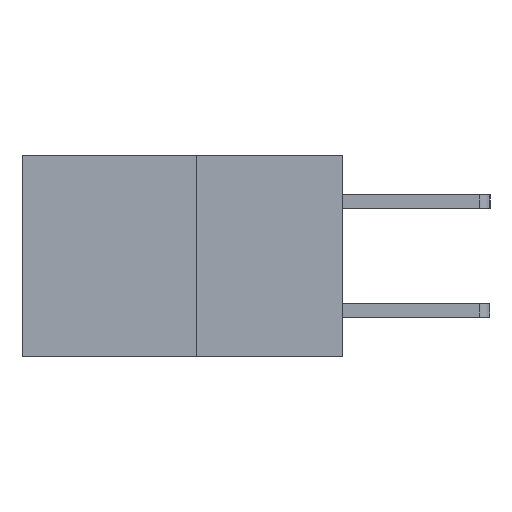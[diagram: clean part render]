
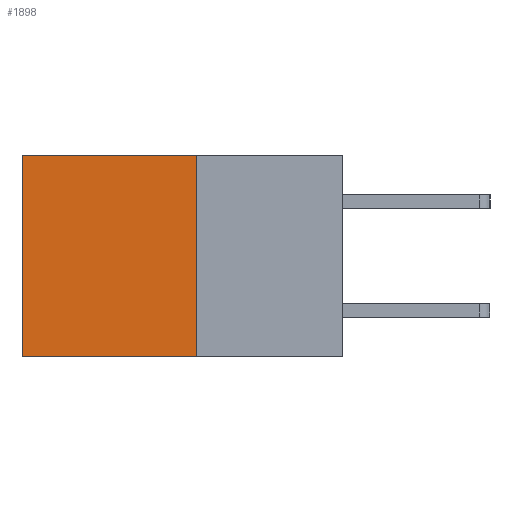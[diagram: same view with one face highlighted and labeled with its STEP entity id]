
A CAD part, left-side view. The second image highlights one B-rep face of the part: STEP entity #1898.
In plain terms, the highlighted planar face has unit normal (-1, 0, 0).
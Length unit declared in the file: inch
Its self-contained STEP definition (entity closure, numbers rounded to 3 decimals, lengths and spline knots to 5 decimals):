
#187 = EDGE_CURVE ( 'NONE', #7900, #6664, #8175, .T. ) ;
#566 = CARTESIAN_POINT ( 'NONE',  ( 0.277, 0.59, -0.37 ) ) ;
#684 = EDGE_LOOP ( 'NONE', ( #6578, #10015, #6638, #6753 ) ) ;
#1254 = CARTESIAN_POINT ( 'NONE',  ( 0.277, 0.59, 0. ) ) ;
#1315 = AXIS2_PLACEMENT_3D ( 'NONE', #9299, #9700, #7021 ) ;
#1421 = DIRECTION ( 'NONE',  ( 0., 0., -1. ) ) ;
#1898 = ADVANCED_FACE ( 'NONE', ( #9473 ), #5515, .F. ) ;
#1937 = DIRECTION ( 'NONE',  ( 0., 1., 0. ) ) ;
#2011 = CARTESIAN_POINT ( 'NONE',  ( 0.277, 0.59, -0.37 ) ) ;
#2542 = CARTESIAN_POINT ( 'NONE',  ( 0.277, 0.27, -0.37 ) ) ;
#2615 = LINE ( 'NONE', #566, #10346 ) ;
#2878 = CARTESIAN_POINT ( 'NONE',  ( 0.277, 0.27, 0. ) ) ;
#3137 = VECTOR ( 'NONE', #6861, 39.37008 ) ;
#3400 = CARTESIAN_POINT ( 'NONE',  ( 0.277, 0.27, -0.37 ) ) ;
#3517 = VERTEX_POINT ( 'NONE', #8911 ) ;
#4864 = EDGE_CURVE ( 'NONE', #7900, #3517, #5909, .T. ) ;
#5427 = DIRECTION ( 'NONE',  ( 0., 0., -1. ) ) ;
#5515 = PLANE ( 'NONE',  #1315 ) ;
#5665 = VECTOR ( 'NONE', #5427, 39.37008 ) ;
#5799 = VERTEX_POINT ( 'NONE', #2011 ) ;
#5909 = LINE ( 'NONE', #3400, #5665 ) ;
#6578 = ORIENTED_EDGE ( 'NONE', *, *, #8843, .T. ) ;
#6638 = ORIENTED_EDGE ( 'NONE', *, *, #4864, .F. ) ;
#6664 = VERTEX_POINT ( 'NONE', #1254 ) ;
#6753 = ORIENTED_EDGE ( 'NONE', *, *, #187, .T. ) ;
#6813 = EDGE_CURVE ( 'NONE', #3517, #5799, #9397, .T. ) ;
#6861 = DIRECTION ( 'NONE',  ( 0., 1., 0. ) ) ;
#7021 = DIRECTION ( 'NONE',  ( 0., 0., -1. ) ) ;
#7900 = VERTEX_POINT ( 'NONE', #8643 ) ;
#8175 = LINE ( 'NONE', #2878, #9822 ) ;
#8643 = CARTESIAN_POINT ( 'NONE',  ( 0.277, 0.27, 0. ) ) ;
#8843 = EDGE_CURVE ( 'NONE', #6664, #5799, #2615, .T. ) ;
#8911 = CARTESIAN_POINT ( 'NONE',  ( 0.277, 0.27, -0.37 ) ) ;
#9299 = CARTESIAN_POINT ( 'NONE',  ( 0.277, 0.27, -0.37 ) ) ;
#9397 = LINE ( 'NONE', #2542, #3137 ) ;
#9473 = FACE_OUTER_BOUND ( 'NONE', #684, .T. ) ;
#9700 = DIRECTION ( 'NONE',  ( 1., 0., 0. ) ) ;
#9822 = VECTOR ( 'NONE', #1937, 39.37008 ) ;
#10015 = ORIENTED_EDGE ( 'NONE', *, *, #6813, .F. ) ;
#10346 = VECTOR ( 'NONE', #1421, 39.37008 ) ;
